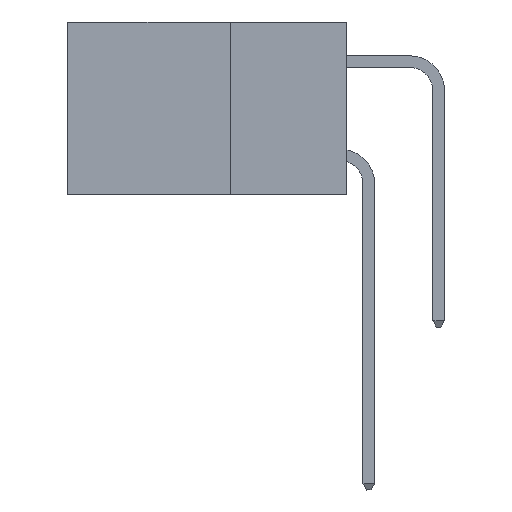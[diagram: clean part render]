
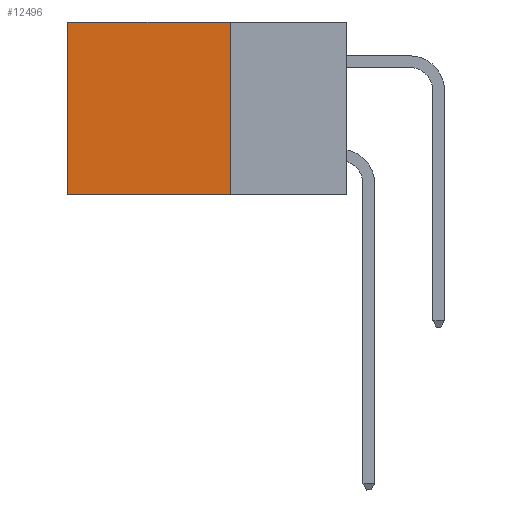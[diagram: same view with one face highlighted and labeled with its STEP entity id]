
A CAD part, left-side view. The second image highlights one B-rep face of the part: STEP entity #12496.
In plain terms, the highlighted planar face has unit normal (-1, 0, 0).
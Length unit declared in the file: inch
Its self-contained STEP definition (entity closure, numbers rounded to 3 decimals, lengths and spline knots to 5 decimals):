
#494 = CARTESIAN_POINT ( 'NONE',  ( 0.2875, 0.6, 0. ) ) ;
#1019 = FACE_OUTER_BOUND ( 'NONE', #17562, .T. ) ;
#1124 = VERTEX_POINT ( 'NONE', #8594 ) ;
#1687 = CARTESIAN_POINT ( 'NONE',  ( 0.2875, 0.25, 0. ) ) ;
#2919 = CARTESIAN_POINT ( 'NONE',  ( 0.2875, 0.6, 0. ) ) ;
#3326 = CARTESIAN_POINT ( 'NONE',  ( 0.2875, 0.6, -0.37 ) ) ;
#3759 = DIRECTION ( 'NONE',  ( 0., 1., 0. ) ) ;
#5137 = VECTOR ( 'NONE', #3759, 39.37008 ) ;
#5901 = VERTEX_POINT ( 'NONE', #11213 ) ;
#6010 = ORIENTED_EDGE ( 'NONE', *, *, #21614, .T. ) ;
#6777 = AXIS2_PLACEMENT_3D ( 'NONE', #11833, #8671, #23831 ) ;
#6857 = EDGE_CURVE ( 'NONE', #13264, #19589, #12200, .T. ) ;
#6905 = VECTOR ( 'NONE', #21524, 39.37008 ) ;
#8118 = EDGE_CURVE ( 'NONE', #1124, #5901, #13009, .T. ) ;
#8594 = CARTESIAN_POINT ( 'NONE',  ( 0.2875, 0.25, 0. ) ) ;
#8671 = DIRECTION ( 'NONE',  ( 1., 0., 0. ) ) ;
#10379 = VECTOR ( 'NONE', #12612, 39.37008 ) ;
#11213 = CARTESIAN_POINT ( 'NONE',  ( 0.2875, 0.25, -0.37 ) ) ;
#11833 = CARTESIAN_POINT ( 'NONE',  ( 0.2875, 0.25, 0. ) ) ;
#12192 = LINE ( 'NONE', #14903, #5137 ) ;
#12200 = LINE ( 'NONE', #2919, #6905 ) ;
#12443 = ORIENTED_EDGE ( 'NONE', *, *, #12652, .F. ) ;
#12496 = ADVANCED_FACE ( 'NONE', ( #1019 ), #19209, .F. ) ;
#12612 = DIRECTION ( 'NONE',  ( 0., 0., -1. ) ) ;
#12652 = EDGE_CURVE ( 'NONE', #5901, #19589, #12192, .T. ) ;
#13009 = LINE ( 'NONE', #1687, #10379 ) ;
#13144 = CARTESIAN_POINT ( 'NONE',  ( 0.2875, 0.25, 0. ) ) ;
#13171 = VECTOR ( 'NONE', #22664, 39.37008 ) ;
#13264 = VERTEX_POINT ( 'NONE', #494 ) ;
#14903 = CARTESIAN_POINT ( 'NONE',  ( 0.2875, 0.25, -0.37 ) ) ;
#16150 = ORIENTED_EDGE ( 'NONE', *, *, #6857, .T. ) ;
#17562 = EDGE_LOOP ( 'NONE', ( #16150, #12443, #23761, #6010 ) ) ;
#19209 = PLANE ( 'NONE',  #6777 ) ;
#19589 = VERTEX_POINT ( 'NONE', #3326 ) ;
#19591 = LINE ( 'NONE', #13144, #13171 ) ;
#21524 = DIRECTION ( 'NONE',  ( 0., 0., -1. ) ) ;
#21614 = EDGE_CURVE ( 'NONE', #1124, #13264, #19591, .T. ) ;
#22664 = DIRECTION ( 'NONE',  ( 0., 1., 0. ) ) ;
#23761 = ORIENTED_EDGE ( 'NONE', *, *, #8118, .F. ) ;
#23831 = DIRECTION ( 'NONE',  ( 0., 0., -1. ) ) ;
